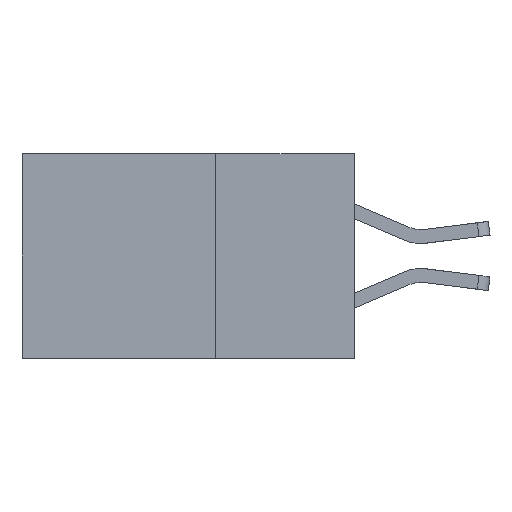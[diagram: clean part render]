
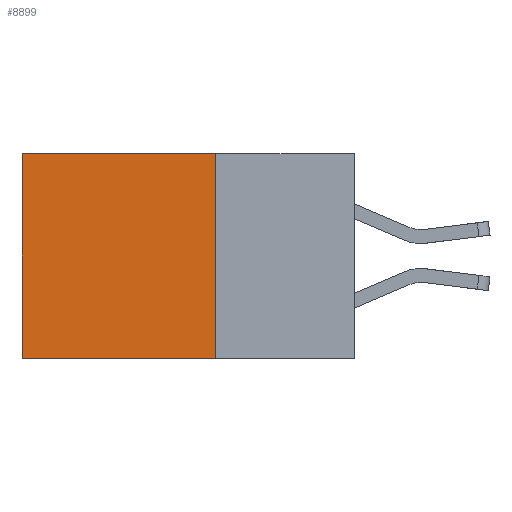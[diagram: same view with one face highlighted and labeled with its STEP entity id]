
A CAD part, left-side view. The second image highlights one B-rep face of the part: STEP entity #8899.
In plain terms, the highlighted planar face has unit normal (-1, 0, 0).
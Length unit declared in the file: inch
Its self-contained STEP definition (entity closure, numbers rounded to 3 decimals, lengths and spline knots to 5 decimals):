
#497 = EDGE_CURVE ( 'NONE', #7725, #8240, #4833, .T. ) ;
#942 = PLANE ( 'NONE',  #6934 ) ;
#1076 = VERTEX_POINT ( 'NONE', #6108 ) ;
#1736 = EDGE_CURVE ( 'NONE', #1744, #8240, #2719, .T. ) ;
#1744 = VERTEX_POINT ( 'NONE', #3247 ) ;
#2189 = LINE ( 'NONE', #6201, #5118 ) ;
#2337 = DIRECTION ( 'NONE',  ( 0., 1., 0. ) ) ;
#2383 = FACE_OUTER_BOUND ( 'NONE', #5284, .T. ) ;
#2385 = CARTESIAN_POINT ( 'NONE',  ( 0.298, 0.25, 0. ) ) ;
#2551 = ORIENTED_EDGE ( 'NONE', *, *, #497, .F. ) ;
#2719 = LINE ( 'NONE', #6977, #5982 ) ;
#3247 = CARTESIAN_POINT ( 'NONE',  ( 0.298, 0.6, 0. ) ) ;
#3321 = ORIENTED_EDGE ( 'NONE', *, *, #4385, .T. ) ;
#3581 = LINE ( 'NONE', #7672, #6844 ) ;
#3916 = CARTESIAN_POINT ( 'NONE',  ( 0.298, 0.25, -0.37 ) ) ;
#4385 = EDGE_CURVE ( 'NONE', #1076, #1744, #2189, .T. ) ;
#4529 = CARTESIAN_POINT ( 'NONE',  ( 0.298, 0.6, -0.37 ) ) ;
#4833 = LINE ( 'NONE', #3916, #5522 ) ;
#5118 = VECTOR ( 'NONE', #6235, 39.37008 ) ;
#5216 = EDGE_CURVE ( 'NONE', #1076, #7725, #3581, .T. ) ;
#5284 = EDGE_LOOP ( 'NONE', ( #6310, #2551, #7464, #3321 ) ) ;
#5522 = VECTOR ( 'NONE', #2337, 39.37008 ) ;
#5535 = DIRECTION ( 'NONE',  ( 0., 0., -1. ) ) ;
#5982 = VECTOR ( 'NONE', #5535, 39.37008 ) ;
#6108 = CARTESIAN_POINT ( 'NONE',  ( 0.298, 0.25, 0. ) ) ;
#6201 = CARTESIAN_POINT ( 'NONE',  ( 0.298, 0.25, 0. ) ) ;
#6235 = DIRECTION ( 'NONE',  ( 0., 1., 0. ) ) ;
#6310 = ORIENTED_EDGE ( 'NONE', *, *, #1736, .T. ) ;
#6844 = VECTOR ( 'NONE', #7640, 39.37008 ) ;
#6934 = AXIS2_PLACEMENT_3D ( 'NONE', #2385, #8370, #9119 ) ;
#6977 = CARTESIAN_POINT ( 'NONE',  ( 0.298, 0.6, 0. ) ) ;
#7464 = ORIENTED_EDGE ( 'NONE', *, *, #5216, .F. ) ;
#7640 = DIRECTION ( 'NONE',  ( 0., 0., -1. ) ) ;
#7672 = CARTESIAN_POINT ( 'NONE',  ( 0.298, 0.25, 0. ) ) ;
#7725 = VERTEX_POINT ( 'NONE', #7818 ) ;
#7818 = CARTESIAN_POINT ( 'NONE',  ( 0.298, 0.25, -0.37 ) ) ;
#8240 = VERTEX_POINT ( 'NONE', #4529 ) ;
#8370 = DIRECTION ( 'NONE',  ( 1., 0., 0. ) ) ;
#8899 = ADVANCED_FACE ( 'NONE', ( #2383 ), #942, .F. ) ;
#9119 = DIRECTION ( 'NONE',  ( 0., 0., -1. ) ) ;
